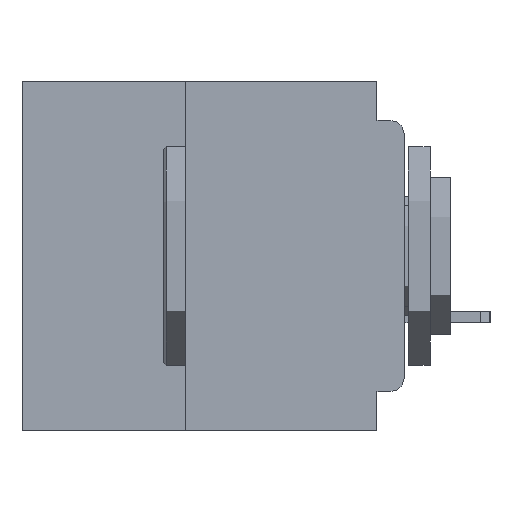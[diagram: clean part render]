
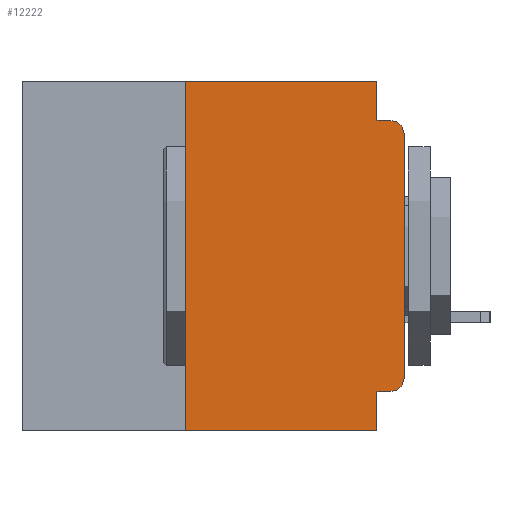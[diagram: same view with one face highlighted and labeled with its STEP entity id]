
A CAD part, left-side view. The second image highlights one B-rep face of the part: STEP entity #12222.
In plain terms, the highlighted planar face has unit normal (-1, 0, 0).
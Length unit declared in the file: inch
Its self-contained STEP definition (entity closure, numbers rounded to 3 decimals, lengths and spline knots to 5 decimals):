
#116 = CIRCLE ( 'NONE', #23988, 0.015 ) ;
#214 = CARTESIAN_POINT ( 'NONE',  ( 0., 0.25, 0. ) ) ;
#1722 = AXIS2_PLACEMENT_3D ( 'NONE', #35415, #20268, #46888 ) ;
#2547 = DIRECTION ( 'NONE',  ( 0., 0., 1. ) ) ;
#2867 = CARTESIAN_POINT ( 'NONE',  ( 0., 0.031, -0.4 ) ) ;
#4876 = VERTEX_POINT ( 'NONE', #35193 ) ;
#5082 = DIRECTION ( 'NONE',  ( 0., 0., -1. ) ) ;
#5785 = EDGE_CURVE ( 'NONE', #29151, #28443, #14079, .T. ) ;
#5928 = CARTESIAN_POINT ( 'NONE',  ( 0., 0.031, -0.045 ) ) ;
#6265 = CARTESIAN_POINT ( 'NONE',  ( 0., 0.437, -0.4 ) ) ;
#7020 = FACE_OUTER_BOUND ( 'NONE', #27674, .T. ) ;
#7025 = CARTESIAN_POINT ( 'NONE',  ( 0., 0., -0.045 ) ) ;
#7390 = CARTESIAN_POINT ( 'NONE',  ( 0., 0.015, -0.045 ) ) ;
#8377 = EDGE_CURVE ( 'NONE', #4876, #46365, #10456, .T. ) ;
#9102 = VECTOR ( 'NONE', #10917, 39.37008 ) ;
#10456 = LINE ( 'NONE', #24160, #20571 ) ;
#10595 = CARTESIAN_POINT ( 'NONE',  ( 0., 0., -0.34 ) ) ;
#10917 = DIRECTION ( 'NONE',  ( 0., -1., 0. ) ) ;
#10930 = LINE ( 'NONE', #12682, #30062 ) ;
#11200 = CARTESIAN_POINT ( 'NONE',  ( 0., 0.015, -0.34 ) ) ;
#11257 = ORIENTED_EDGE ( 'NONE', *, *, #41058, .T. ) ;
#11344 = EDGE_CURVE ( 'NONE', #40362, #28188, #14934, .T. ) ;
#12082 = CARTESIAN_POINT ( 'NONE',  ( 0., 0.015, -0.355 ) ) ;
#12222 = ADVANCED_FACE ( 'NONE', ( #7020 ), #43092, .F. ) ;
#12469 = ORIENTED_EDGE ( 'NONE', *, *, #31824, .T. ) ;
#12521 = ORIENTED_EDGE ( 'NONE', *, *, #23130, .F. ) ;
#12682 = CARTESIAN_POINT ( 'NONE',  ( 0., 0., 0. ) ) ;
#12870 = DIRECTION ( 'NONE',  ( 0., 0., -1. ) ) ;
#13274 = CARTESIAN_POINT ( 'NONE',  ( 0., 0.015, -0.06 ) ) ;
#13779 = ORIENTED_EDGE ( 'NONE', *, *, #8377, .F. ) ;
#13865 = CARTESIAN_POINT ( 'NONE',  ( 0., 0., -0.355 ) ) ;
#13870 = DIRECTION ( 'NONE',  ( 0., -1., 0. ) ) ;
#14079 = LINE ( 'NONE', #29376, #22969 ) ;
#14109 = ORIENTED_EDGE ( 'NONE', *, *, #43714, .F. ) ;
#14922 = ORIENTED_EDGE ( 'NONE', *, *, #5785, .F. ) ;
#14934 = CIRCLE ( 'NONE', #31231, 0.015 ) ;
#15053 = DIRECTION ( 'NONE',  ( 0., 0., -1. ) ) ;
#15528 = ORIENTED_EDGE ( 'NONE', *, *, #34895, .T. ) ;
#16166 = VERTEX_POINT ( 'NONE', #34538 ) ;
#16499 = DIRECTION ( 'NONE',  ( 0., 0., 1. ) ) ;
#16535 = CARTESIAN_POINT ( 'NONE',  ( 0., 0.437, 0. ) ) ;
#17086 = DIRECTION ( 'NONE',  ( 0., 0., -1. ) ) ;
#17151 = ORIENTED_EDGE ( 'NONE', *, *, #32416, .F. ) ;
#18024 = ORIENTED_EDGE ( 'NONE', *, *, #39445, .F. ) ;
#18117 = ORIENTED_EDGE ( 'NONE', *, *, #11344, .T. ) ;
#20268 = DIRECTION ( 'NONE',  ( 1., 0., 0. ) ) ;
#20571 = VECTOR ( 'NONE', #5082, 39.37008 ) ;
#21129 = CARTESIAN_POINT ( 'NONE',  ( 0., 0.031, -0.355 ) ) ;
#22969 = VECTOR ( 'NONE', #2547, 39.37008 ) ;
#23130 = EDGE_CURVE ( 'NONE', #46365, #31557, #30658, .T. ) ;
#23462 = LINE ( 'NONE', #43324, #32497 ) ;
#23988 = AXIS2_PLACEMENT_3D ( 'NONE', #13274, #39909, #17086 ) ;
#24160 = CARTESIAN_POINT ( 'NONE',  ( 0., 0.031, 0. ) ) ;
#24398 = LINE ( 'NONE', #6265, #44652 ) ;
#25412 = VECTOR ( 'NONE', #33032, 39.37008 ) ;
#26817 = VECTOR ( 'NONE', #39357, 39.37008 ) ;
#27674 = EDGE_LOOP ( 'NONE', ( #11257, #12469, #12521, #13779, #14109, #14922, #15528, #17151, #18024, #18117 ) ) ;
#28188 = VERTEX_POINT ( 'NONE', #10595 ) ;
#28443 = VERTEX_POINT ( 'NONE', #214 ) ;
#29151 = VERTEX_POINT ( 'NONE', #35470 ) ;
#29376 = CARTESIAN_POINT ( 'NONE',  ( 0., 0.25, -0.4 ) ) ;
#30062 = VECTOR ( 'NONE', #16499, 39.37008 ) ;
#30658 = LINE ( 'NONE', #7025, #9102 ) ;
#31231 = AXIS2_PLACEMENT_3D ( 'NONE', #11200, #37854, #15053 ) ;
#31557 = VERTEX_POINT ( 'NONE', #7390 ) ;
#31824 = EDGE_CURVE ( 'NONE', #16166, #31557, #116, .T. ) ;
#32416 = EDGE_CURVE ( 'NONE', #47092, #47232, #23462, .T. ) ;
#32497 = VECTOR ( 'NONE', #12870, 39.37008 ) ;
#33032 = DIRECTION ( 'NONE',  ( 0., 1., 0. ) ) ;
#34538 = CARTESIAN_POINT ( 'NONE',  ( 0., 0., -0.06 ) ) ;
#34895 = EDGE_CURVE ( 'NONE', #29151, #47232, #24398, .T. ) ;
#35193 = CARTESIAN_POINT ( 'NONE',  ( 0., 0.031, 0. ) ) ;
#35415 = CARTESIAN_POINT ( 'NONE',  ( 0., 0.437, 0. ) ) ;
#35470 = CARTESIAN_POINT ( 'NONE',  ( 0., 0.25, -0.4 ) ) ;
#37854 = DIRECTION ( 'NONE',  ( -1., 0., 0. ) ) ;
#39357 = DIRECTION ( 'NONE',  ( 0., -1., 0. ) ) ;
#39445 = EDGE_CURVE ( 'NONE', #40362, #47092, #48009, .T. ) ;
#39909 = DIRECTION ( 'NONE',  ( -1., 0., 0. ) ) ;
#40362 = VERTEX_POINT ( 'NONE', #12082 ) ;
#41058 = EDGE_CURVE ( 'NONE', #28188, #16166, #10930, .T. ) ;
#43092 = PLANE ( 'NONE',  #1722 ) ;
#43324 = CARTESIAN_POINT ( 'NONE',  ( 0., 0.031, -0.4 ) ) ;
#43714 = EDGE_CURVE ( 'NONE', #28443, #4876, #44662, .T. ) ;
#44652 = VECTOR ( 'NONE', #13870, 39.37008 ) ;
#44662 = LINE ( 'NONE', #16535, #26817 ) ;
#46365 = VERTEX_POINT ( 'NONE', #5928 ) ;
#46888 = DIRECTION ( 'NONE',  ( 0., 0., -1. ) ) ;
#47092 = VERTEX_POINT ( 'NONE', #21129 ) ;
#47232 = VERTEX_POINT ( 'NONE', #2867 ) ;
#48009 = LINE ( 'NONE', #13865, #25412 ) ;
